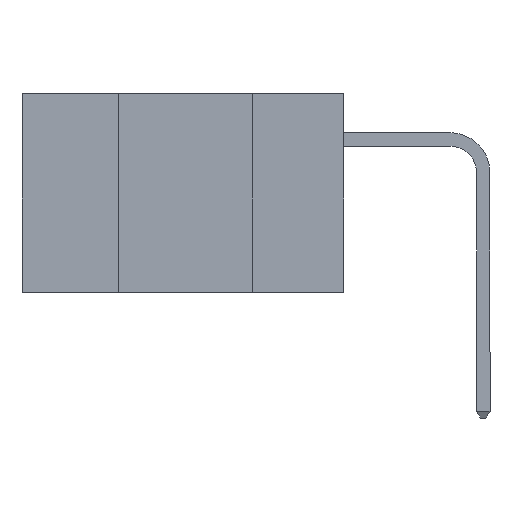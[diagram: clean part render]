
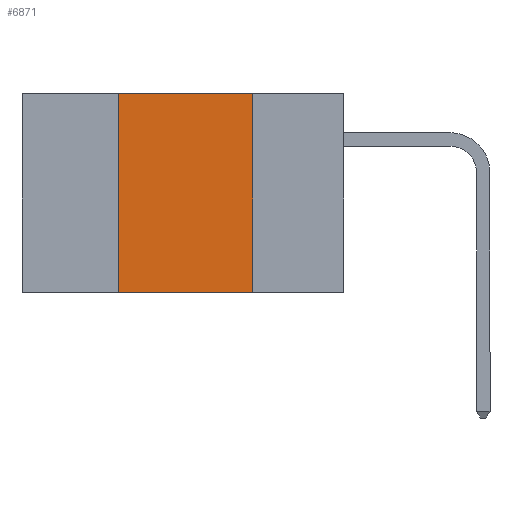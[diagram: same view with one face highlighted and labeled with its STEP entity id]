
A CAD part, left-side view. The second image highlights one B-rep face of the part: STEP entity #6871.
In plain terms, the highlighted planar face has unit normal (-1, 0, 0).
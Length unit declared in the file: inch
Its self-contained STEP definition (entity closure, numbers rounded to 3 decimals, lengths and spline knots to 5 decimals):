
#434 = CARTESIAN_POINT ( 'NONE',  ( 0., 0.17, 0. ) ) ;
#614 = ORIENTED_EDGE ( 'NONE', *, *, #3999, .F. ) ;
#719 = ORIENTED_EDGE ( 'NONE', *, *, #2678, .T. ) ;
#800 = DIRECTION ( 'NONE',  ( 0., 0., -1. ) ) ;
#821 = DIRECTION ( 'NONE',  ( 1., 0., 0. ) ) ;
#836 = CARTESIAN_POINT ( 'NONE',  ( 0., 0.6, 0. ) ) ;
#860 = PLANE ( 'NONE',  #1390 ) ;
#902 = EDGE_CURVE ( 'NONE', #2131, #3397, #3921, .T. ) ;
#1390 = AXIS2_PLACEMENT_3D ( 'NONE', #836, #821, #800 ) ;
#1563 = ORIENTED_EDGE ( 'NONE', *, *, #902, .F. ) ;
#2131 = VERTEX_POINT ( 'NONE', #11152 ) ;
#2678 = EDGE_CURVE ( 'NONE', #2131, #5421, #4689, .T. ) ;
#3256 = CARTESIAN_POINT ( 'NONE',  ( 0., 0.17, -0.37 ) ) ;
#3397 = VERTEX_POINT ( 'NONE', #7853 ) ;
#3557 = LINE ( 'NONE', #434, #5340 ) ;
#3921 = LINE ( 'NONE', #10501, #8125 ) ;
#3999 = EDGE_CURVE ( 'NONE', #6060, #5421, #3557, .T. ) ;
#4596 = DIRECTION ( 'NONE',  ( 0., 0., -1. ) ) ;
#4689 = LINE ( 'NONE', #6599, #11016 ) ;
#5340 = VECTOR ( 'NONE', #4596, 39.37008 ) ;
#5421 = VERTEX_POINT ( 'NONE', #3256 ) ;
#6060 = VERTEX_POINT ( 'NONE', #9103 ) ;
#6084 = EDGE_CURVE ( 'NONE', #3397, #6060, #10717, .T. ) ;
#6599 = CARTESIAN_POINT ( 'NONE',  ( 0., 0.6, -0.37 ) ) ;
#6613 = VECTOR ( 'NONE', #8939, 39.37008 ) ;
#6871 = ADVANCED_FACE ( 'NONE', ( #11084 ), #860, .F. ) ;
#7610 = EDGE_LOOP ( 'NONE', ( #614, #8985, #1563, #719 ) ) ;
#7853 = CARTESIAN_POINT ( 'NONE',  ( 0., 0.42, 0. ) ) ;
#8125 = VECTOR ( 'NONE', #10793, 39.37008 ) ;
#8939 = DIRECTION ( 'NONE',  ( 0., -1., 0. ) ) ;
#8985 = ORIENTED_EDGE ( 'NONE', *, *, #6084, .F. ) ;
#9103 = CARTESIAN_POINT ( 'NONE',  ( 0., 0.17, 0. ) ) ;
#9112 = CARTESIAN_POINT ( 'NONE',  ( 0., 0.6, 0. ) ) ;
#9572 = DIRECTION ( 'NONE',  ( 0., -1., 0. ) ) ;
#10501 = CARTESIAN_POINT ( 'NONE',  ( 0., 0.42, 0. ) ) ;
#10717 = LINE ( 'NONE', #9112, #6613 ) ;
#10793 = DIRECTION ( 'NONE',  ( 0., 0., 1. ) ) ;
#11016 = VECTOR ( 'NONE', #9572, 39.37008 ) ;
#11084 = FACE_OUTER_BOUND ( 'NONE', #7610, .T. ) ;
#11152 = CARTESIAN_POINT ( 'NONE',  ( 0., 0.42, -0.37 ) ) ;
